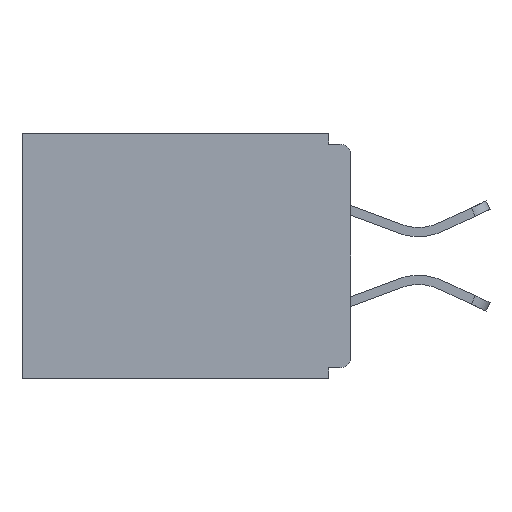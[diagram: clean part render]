
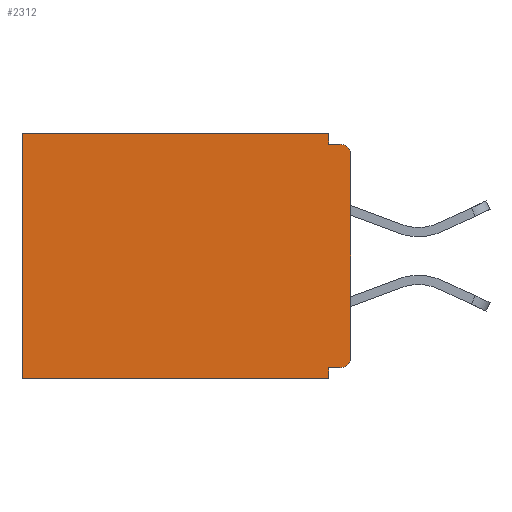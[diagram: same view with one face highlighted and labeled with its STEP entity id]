
A CAD part, left-side view. The second image highlights one B-rep face of the part: STEP entity #2312.
In plain terms, the highlighted planar face has unit normal (-1, 0, 0).
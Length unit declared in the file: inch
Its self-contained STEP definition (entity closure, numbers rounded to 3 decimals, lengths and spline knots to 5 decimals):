
#94 = DIRECTION ( 'NONE',  ( 0., 0., -1. ) ) ;
#144 = CARTESIAN_POINT ( 'NONE',  ( 0.298, 0.015, -0.313 ) ) ;
#290 = FACE_OUTER_BOUND ( 'NONE', #9259, .T. ) ;
#566 = VERTEX_POINT ( 'NONE', #3462 ) ;
#794 = ORIENTED_EDGE ( 'NONE', *, *, #9798, .F. ) ;
#931 = DIRECTION ( 'NONE',  ( 0., 0., -1. ) ) ;
#941 = ORIENTED_EDGE ( 'NONE', *, *, #7081, .T. ) ;
#1707 = CARTESIAN_POINT ( 'NONE',  ( 0.298, 0.031, -0.328 ) ) ;
#1733 = VECTOR ( 'NONE', #8341, 39.37008 ) ;
#1754 = VERTEX_POINT ( 'NONE', #1707 ) ;
#2026 = PLANE ( 'NONE',  #6237 ) ;
#2043 = LINE ( 'NONE', #9231, #4038 ) ;
#2076 = VERTEX_POINT ( 'NONE', #7432 ) ;
#2188 = CARTESIAN_POINT ( 'NONE',  ( 0.298, 0.015, -0.328 ) ) ;
#2234 = CARTESIAN_POINT ( 'NONE',  ( 0.298, 0.031, -0.343 ) ) ;
#2312 = ADVANCED_FACE ( 'NONE', ( #290 ), #2026, .F. ) ;
#2789 = CIRCLE ( 'NONE', #8910, 0.015 ) ;
#2837 = VERTEX_POINT ( 'NONE', #2234 ) ;
#2931 = VECTOR ( 'NONE', #11526, 39.37008 ) ;
#3063 = ORIENTED_EDGE ( 'NONE', *, *, #10062, .F. ) ;
#3241 = CARTESIAN_POINT ( 'NONE',  ( 0.298, 0.031, -0.343 ) ) ;
#3346 = DIRECTION ( 'NONE',  ( 0., 1., 0. ) ) ;
#3429 = CARTESIAN_POINT ( 'NONE',  ( 0.298, 0., -0.03 ) ) ;
#3432 = VERTEX_POINT ( 'NONE', #3429 ) ;
#3462 = CARTESIAN_POINT ( 'NONE',  ( 0.298, 0., -0.313 ) ) ;
#3794 = CARTESIAN_POINT ( 'NONE',  ( 0.298, 0., -0.015 ) ) ;
#4038 = VECTOR ( 'NONE', #11142, 39.37008 ) ;
#4126 = VERTEX_POINT ( 'NONE', #4511 ) ;
#4182 = EDGE_CURVE ( 'NONE', #4126, #8217, #4381, .T. ) ;
#4230 = DIRECTION ( 'NONE',  ( 0., 0., -1. ) ) ;
#4323 = CARTESIAN_POINT ( 'NONE',  ( 0.298, 0.46, 0. ) ) ;
#4381 = LINE ( 'NONE', #3794, #8552 ) ;
#4511 = CARTESIAN_POINT ( 'NONE',  ( 0.298, 0.031, -0.015 ) ) ;
#4628 = LINE ( 'NONE', #7613, #7723 ) ;
#4804 = DIRECTION ( 'NONE',  ( 0., -1., 0. ) ) ;
#4955 = LINE ( 'NONE', #8373, #12356 ) ;
#5098 = CARTESIAN_POINT ( 'NONE',  ( 0.298, 0.015, -0.03 ) ) ;
#5403 = CARTESIAN_POINT ( 'NONE',  ( 0.298, 0.46, -0.343 ) ) ;
#5989 = ORIENTED_EDGE ( 'NONE', *, *, #11248, .F. ) ;
#6036 = CARTESIAN_POINT ( 'NONE',  ( 0.298, 0., 0. ) ) ;
#6237 = AXIS2_PLACEMENT_3D ( 'NONE', #6036, #7845, #931 ) ;
#6257 = DIRECTION ( 'NONE',  ( 0., 0., -1. ) ) ;
#6361 = LINE ( 'NONE', #3241, #1733 ) ;
#6635 = ORIENTED_EDGE ( 'NONE', *, *, #6867, .T. ) ;
#6736 = CARTESIAN_POINT ( 'NONE',  ( 0.298, 0.015, -0.015 ) ) ;
#6867 = EDGE_CURVE ( 'NONE', #3432, #8217, #2789, .T. ) ;
#6917 = DIRECTION ( 'NONE',  ( 0., 1., 0. ) ) ;
#7081 = EDGE_CURVE ( 'NONE', #7721, #566, #9252, .T. ) ;
#7246 = LINE ( 'NONE', #12310, #8169 ) ;
#7432 = CARTESIAN_POINT ( 'NONE',  ( 0.298, 0.031, 0. ) ) ;
#7613 = CARTESIAN_POINT ( 'NONE',  ( 0.298, 0., 0. ) ) ;
#7627 = ORIENTED_EDGE ( 'NONE', *, *, #11740, .T. ) ;
#7721 = VERTEX_POINT ( 'NONE', #2188 ) ;
#7723 = VECTOR ( 'NONE', #6917, 39.37008 ) ;
#7845 = DIRECTION ( 'NONE',  ( 1., 0., 0. ) ) ;
#8169 = VECTOR ( 'NONE', #3346, 39.37008 ) ;
#8217 = VERTEX_POINT ( 'NONE', #6736 ) ;
#8341 = DIRECTION ( 'NONE',  ( 0., 0., -1. ) ) ;
#8356 = ORIENTED_EDGE ( 'NONE', *, *, #4182, .F. ) ;
#8373 = CARTESIAN_POINT ( 'NONE',  ( 0.298, 0., 0. ) ) ;
#8552 = VECTOR ( 'NONE', #4804, 39.37008 ) ;
#8830 = CARTESIAN_POINT ( 'NONE',  ( 0.298, 0.46, 0. ) ) ;
#8910 = AXIS2_PLACEMENT_3D ( 'NONE', #5098, #10044, #4230 ) ;
#8974 = DIRECTION ( 'NONE',  ( -1., 0., 0. ) ) ;
#9231 = CARTESIAN_POINT ( 'NONE',  ( 0.298, 0.031, -0.343 ) ) ;
#9252 = CIRCLE ( 'NONE', #11551, 0.015 ) ;
#9259 = EDGE_LOOP ( 'NONE', ( #6635, #8356, #794, #11360, #7627, #5989, #12727, #9497, #941, #3063 ) ) ;
#9487 = EDGE_CURVE ( 'NONE', #1754, #2837, #2043, .T. ) ;
#9497 = ORIENTED_EDGE ( 'NONE', *, *, #11805, .F. ) ;
#9703 = CARTESIAN_POINT ( 'NONE',  ( 0.298, 0., -0.343 ) ) ;
#9798 = EDGE_CURVE ( 'NONE', #2076, #4126, #6361, .T. ) ;
#10044 = DIRECTION ( 'NONE',  ( -1., 0., 0. ) ) ;
#10062 = EDGE_CURVE ( 'NONE', #3432, #566, #4955, .T. ) ;
#10335 = LINE ( 'NONE', #9703, #2931 ) ;
#10385 = DIRECTION ( 'NONE',  ( 0., 0., -1. ) ) ;
#10469 = LINE ( 'NONE', #4323, #12482 ) ;
#10800 = VERTEX_POINT ( 'NONE', #5403 ) ;
#11142 = DIRECTION ( 'NONE',  ( 0., 0., -1. ) ) ;
#11248 = EDGE_CURVE ( 'NONE', #2837, #10800, #10335, .T. ) ;
#11360 = ORIENTED_EDGE ( 'NONE', *, *, #11421, .T. ) ;
#11421 = EDGE_CURVE ( 'NONE', #2076, #12449, #4628, .T. ) ;
#11526 = DIRECTION ( 'NONE',  ( 0., 1., 0. ) ) ;
#11551 = AXIS2_PLACEMENT_3D ( 'NONE', #144, #8974, #94 ) ;
#11740 = EDGE_CURVE ( 'NONE', #12449, #10800, #10469, .T. ) ;
#11805 = EDGE_CURVE ( 'NONE', #7721, #1754, #7246, .T. ) ;
#12310 = CARTESIAN_POINT ( 'NONE',  ( 0.298, 0., -0.328 ) ) ;
#12356 = VECTOR ( 'NONE', #6257, 39.37008 ) ;
#12449 = VERTEX_POINT ( 'NONE', #8830 ) ;
#12482 = VECTOR ( 'NONE', #10385, 39.37008 ) ;
#12727 = ORIENTED_EDGE ( 'NONE', *, *, #9487, .F. ) ;
